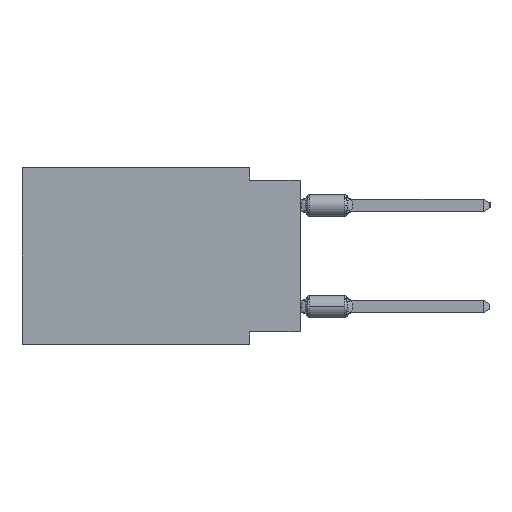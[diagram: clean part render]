
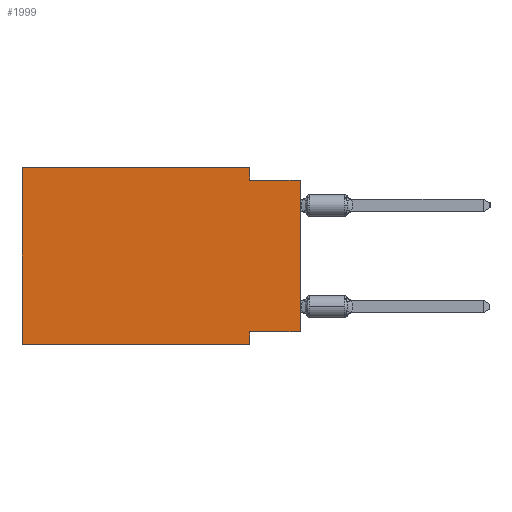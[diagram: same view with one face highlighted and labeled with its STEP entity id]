
A CAD part, left-side view. The second image highlights one B-rep face of the part: STEP entity #1999.
In plain terms, the highlighted planar face has unit normal (-1, 0, 0).
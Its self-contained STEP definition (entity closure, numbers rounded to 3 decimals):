
#5 = DIRECTION ( 'NONE',  ( 0., 0., -1. ) ) ;
#118 = VERTEX_POINT ( 'NONE', #1365 ) ;
#253 = CARTESIAN_POINT ( 'NONE',  ( 0., 13.97, -8.89 ) ) ;
#1069 = CARTESIAN_POINT ( 'NONE',  ( 0., 2.54, -8.255 ) ) ;
#1168 = VECTOR ( 'NONE', #4132, 1000. ) ;
#1365 = CARTESIAN_POINT ( 'NONE',  ( 0., 2.54, 0. ) ) ;
#1999 = ADVANCED_FACE ( 'NONE', ( #7815 ), #3633, .F. ) ;
#2396 = ORIENTED_EDGE ( 'NONE', *, *, #18113, .T. ) ;
#2775 = CARTESIAN_POINT ( 'NONE',  ( 0., 13.97, 0. ) ) ;
#3125 = VERTEX_POINT ( 'NONE', #253 ) ;
#3320 = VECTOR ( 'NONE', #5, 1000. ) ;
#3633 = PLANE ( 'NONE',  #25900 ) ;
#3782 = CARTESIAN_POINT ( 'NONE',  ( 0., 13.97, 0. ) ) ;
#4132 = DIRECTION ( 'NONE',  ( 0., 0., 1. ) ) ;
#4173 = DIRECTION ( 'NONE',  ( 0., -1., 0. ) ) ;
#4465 = CARTESIAN_POINT ( 'NONE',  ( 0., 13.97, 0. ) ) ;
#4628 = LINE ( 'NONE', #16342, #3320 ) ;
#4750 = VERTEX_POINT ( 'NONE', #11826 ) ;
#4870 = DIRECTION ( 'NONE',  ( 0., -1., 0. ) ) ;
#4987 = CARTESIAN_POINT ( 'NONE',  ( 0., 2.54, -8.89 ) ) ;
#5494 = DIRECTION ( 'NONE',  ( 0., 0., -1. ) ) ;
#5610 = VECTOR ( 'NONE', #4173, 1000. ) ;
#5650 = VERTEX_POINT ( 'NONE', #29193 ) ;
#7337 = LINE ( 'NONE', #19350, #15598 ) ;
#7561 = LINE ( 'NONE', #2775, #15625 ) ;
#7815 = FACE_OUTER_BOUND ( 'NONE', #22051, .T. ) ;
#7937 = EDGE_CURVE ( 'NONE', #4750, #18063, #13845, .T. ) ;
#8098 = CARTESIAN_POINT ( 'NONE',  ( 0., 0., -8.255 ) ) ;
#8724 = EDGE_CURVE ( 'NONE', #8967, #18063, #15745, .T. ) ;
#8967 = VERTEX_POINT ( 'NONE', #10629 ) ;
#9145 = DIRECTION ( 'NONE',  ( 0., 0., -1. ) ) ;
#9170 = CARTESIAN_POINT ( 'NONE',  ( 0., 0., -0.635 ) ) ;
#9708 = DIRECTION ( 'NONE',  ( 0., 0., 1. ) ) ;
#10629 = CARTESIAN_POINT ( 'NONE',  ( 0., 2.54, -0.635 ) ) ;
#11826 = CARTESIAN_POINT ( 'NONE',  ( 0., 0., -8.255 ) ) ;
#12092 = DIRECTION ( 'NONE',  ( 0., -1., 0. ) ) ;
#12737 = DIRECTION ( 'NONE',  ( 1., 0., 0. ) ) ;
#12811 = ORIENTED_EDGE ( 'NONE', *, *, #20149, .F. ) ;
#13845 = LINE ( 'NONE', #29721, #1168 ) ;
#15598 = VECTOR ( 'NONE', #4870, 1000. ) ;
#15625 = VECTOR ( 'NONE', #9708, 1000. ) ;
#15745 = LINE ( 'NONE', #20975, #5610 ) ;
#15980 = ORIENTED_EDGE ( 'NONE', *, *, #8724, .F. ) ;
#16246 = LINE ( 'NONE', #4987, #23642 ) ;
#16342 = CARTESIAN_POINT ( 'NONE',  ( 0., 2.54, 0. ) ) ;
#16437 = VECTOR ( 'NONE', #12092, 1000. ) ;
#16630 = ORIENTED_EDGE ( 'NONE', *, *, #29881, .F. ) ;
#18063 = VERTEX_POINT ( 'NONE', #9170 ) ;
#18113 = EDGE_CURVE ( 'NONE', #3125, #5650, #18564, .T. ) ;
#18264 = EDGE_CURVE ( 'NONE', #4750, #21516, #29195, .T. ) ;
#18291 = ORIENTED_EDGE ( 'NONE', *, *, #7937, .T. ) ;
#18564 = LINE ( 'NONE', #23352, #16437 ) ;
#18963 = ORIENTED_EDGE ( 'NONE', *, *, #18264, .F. ) ;
#19350 = CARTESIAN_POINT ( 'NONE',  ( 0., 13.97, 0. ) ) ;
#20149 = EDGE_CURVE ( 'NONE', #118, #8967, #4628, .T. ) ;
#20254 = EDGE_CURVE ( 'NONE', #3125, #27607, #7561, .T. ) ;
#20975 = CARTESIAN_POINT ( 'NONE',  ( 0., 0., -0.635 ) ) ;
#21376 = VECTOR ( 'NONE', #28731, 1000. ) ;
#21516 = VERTEX_POINT ( 'NONE', #1069 ) ;
#22051 = EDGE_LOOP ( 'NONE', ( #18291, #15980, #12811, #16630, #27666, #2396, #25655, #18963 ) ) ;
#23352 = CARTESIAN_POINT ( 'NONE',  ( 0., 13.97, -8.89 ) ) ;
#23642 = VECTOR ( 'NONE', #9145, 1000. ) ;
#25037 = EDGE_CURVE ( 'NONE', #21516, #5650, #16246, .T. ) ;
#25655 = ORIENTED_EDGE ( 'NONE', *, *, #25037, .F. ) ;
#25900 = AXIS2_PLACEMENT_3D ( 'NONE', #3782, #12737, #5494 ) ;
#27607 = VERTEX_POINT ( 'NONE', #4465 ) ;
#27666 = ORIENTED_EDGE ( 'NONE', *, *, #20254, .F. ) ;
#28731 = DIRECTION ( 'NONE',  ( 0., 1., 0. ) ) ;
#29193 = CARTESIAN_POINT ( 'NONE',  ( 0., 2.54, -8.89 ) ) ;
#29195 = LINE ( 'NONE', #8098, #21376 ) ;
#29721 = CARTESIAN_POINT ( 'NONE',  ( 0., 0., 0. ) ) ;
#29881 = EDGE_CURVE ( 'NONE', #27607, #118, #7337, .T. ) ;
